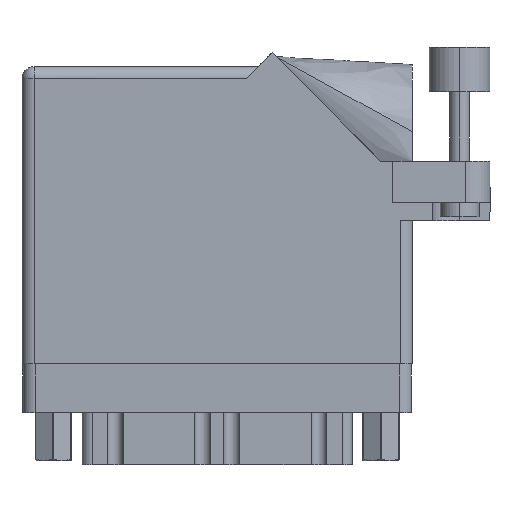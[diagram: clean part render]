
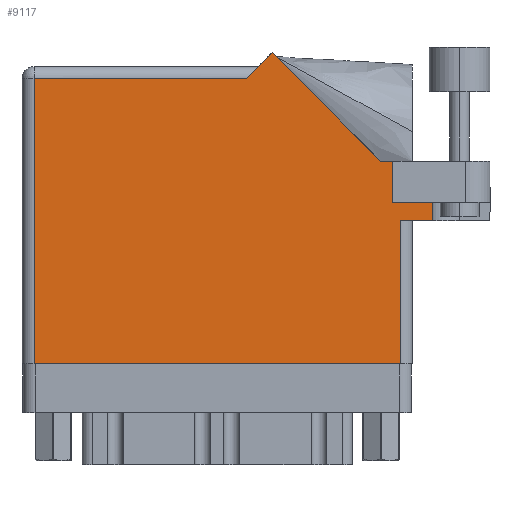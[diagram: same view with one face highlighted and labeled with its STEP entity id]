
A CAD part, front view. The second image highlights one B-rep face of the part: STEP entity #9117.
In plain terms, the highlighted face is planar.
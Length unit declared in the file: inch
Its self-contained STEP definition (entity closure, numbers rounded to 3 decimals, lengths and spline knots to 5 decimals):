
#818 = ORIENTED_EDGE ( 'NONE', *, *, #22465, .T. ) ;
#1750 = FACE_OUTER_BOUND ( 'NONE', #42645, .T. ) ;
#2393 = ORIENTED_EDGE ( 'NONE', *, *, #38100, .T. ) ;
#2926 = CARTESIAN_POINT ( 'NONE',  ( 1.948, 0.737, 0. ) ) ;
#2951 = VERTEX_POINT ( 'NONE', #8101 ) ;
#3372 = LINE ( 'NONE', #7256, #15728 ) ;
#3553 = VERTEX_POINT ( 'NONE', #5469 ) ;
#4420 = EDGE_CURVE ( 'NONE', #41821, #39390, #45638, .T. ) ;
#4458 = VECTOR ( 'NONE', #14354, 39.37008 ) ;
#4657 = CARTESIAN_POINT ( 'NONE',  ( 1.948, 0.737, 0. ) ) ;
#5469 = CARTESIAN_POINT ( 'NONE',  ( 1.91, 1.044, 0. ) ) ;
#5894 = EDGE_CURVE ( 'NONE', #24970, #6006, #18654, .T. ) ;
#6006 = VERTEX_POINT ( 'NONE', #43447 ) ;
#6350 = EDGE_CURVE ( 'NONE', #17928, #39390, #37584, .T. ) ;
#6385 = VECTOR ( 'NONE', #17663, 39.37008 ) ;
#7256 = CARTESIAN_POINT ( 'NONE',  ( 1.84442, 1.044, 0. ) ) ;
#7576 = LINE ( 'NONE', #33860, #27539 ) ;
#8101 = CARTESIAN_POINT ( 'NONE',  ( 1.91, 0.831, 0. ) ) ;
#8550 = ORIENTED_EDGE ( 'NONE', *, *, #29439, .T. ) ;
#9117 = ADVANCED_FACE ( 'NONE', ( #1750 ), #26861, .F. ) ;
#9254 = CARTESIAN_POINT ( 'NONE',  ( 0., 1.468, 0. ) ) ;
#9291 = CARTESIAN_POINT ( 'NONE',  ( 1.91, 0.831, 0. ) ) ;
#10376 = CARTESIAN_POINT ( 'NONE',  ( 2.1115, 0.737, 0. ) ) ;
#10436 = CARTESIAN_POINT ( 'NONE',  ( 1.84442, 1.044, 0. ) ) ;
#13800 = VECTOR ( 'NONE', #30621, 39.37008 ) ;
#14354 = DIRECTION ( 'NONE',  ( -0.707, -0.707, 0. ) ) ;
#15728 = VECTOR ( 'NONE', #18330, 39.37008 ) ;
#16758 = CARTESIAN_POINT ( 'NONE',  ( 0.062, 1.468, 0. ) ) ;
#17663 = DIRECTION ( 'NONE',  ( 0., 1., 0. ) ) ;
#17928 = VERTEX_POINT ( 'NONE', #23054 ) ;
#18197 = LINE ( 'NONE', #39715, #4458 ) ;
#18330 = DIRECTION ( 'NONE',  ( -0.707, 0.707, 0. ) ) ;
#18363 = VECTOR ( 'NONE', #45810, 39.37008 ) ;
#18483 = ORIENTED_EDGE ( 'NONE', *, *, #25661, .T. ) ;
#18531 = ORIENTED_EDGE ( 'NONE', *, *, #46637, .F. ) ;
#18654 = LINE ( 'NONE', #19109, #40227 ) ;
#19109 = CARTESIAN_POINT ( 'NONE',  ( 0.062, 0., 0. ) ) ;
#19128 = VECTOR ( 'NONE', #41120, 39.37008 ) ;
#19807 = EDGE_CURVE ( 'NONE', #6006, #39702, #22893, .T. ) ;
#20011 = ORIENTED_EDGE ( 'NONE', *, *, #28339, .T. ) ;
#21288 = LINE ( 'NONE', #2926, #6385 ) ;
#22444 = VERTEX_POINT ( 'NONE', #10436 ) ;
#22465 = EDGE_CURVE ( 'NONE', #39702, #41821, #21288, .T. ) ;
#22553 = CARTESIAN_POINT ( 'NONE',  ( 1.155, 1.468, 0. ) ) ;
#22893 = LINE ( 'NONE', #27870, #30892 ) ;
#22985 = DIRECTION ( 'NONE',  ( -1., 0., 0. ) ) ;
#23054 = CARTESIAN_POINT ( 'NONE',  ( 2.1115, 0.831, 0. ) ) ;
#23489 = CARTESIAN_POINT ( 'NONE',  ( 0., 1.53, 0. ) ) ;
#24970 = VERTEX_POINT ( 'NONE', #16758 ) ;
#25661 = EDGE_CURVE ( 'NONE', #22444, #30979, #3372, .T. ) ;
#25955 = VECTOR ( 'NONE', #38731, 39.37008 ) ;
#26861 = PLANE ( 'NONE',  #30449 ) ;
#27112 = LINE ( 'NONE', #9254, #38054 ) ;
#27249 = ORIENTED_EDGE ( 'NONE', *, *, #5894, .T. ) ;
#27539 = VECTOR ( 'NONE', #22985, 39.37008 ) ;
#27870 = CARTESIAN_POINT ( 'NONE',  ( 0., 0., 0. ) ) ;
#28072 = EDGE_CURVE ( 'NONE', #2951, #3553, #42371, .T. ) ;
#28339 = EDGE_CURVE ( 'NONE', #3553, #22444, #7576, .T. ) ;
#29439 = EDGE_CURVE ( 'NONE', #30979, #45031, #18197, .T. ) ;
#30449 = AXIS2_PLACEMENT_3D ( 'NONE', #23489, #45952, #41614 ) ;
#30621 = DIRECTION ( 'NONE',  ( 1., 0., 0. ) ) ;
#30892 = VECTOR ( 'NONE', #42628, 39.37008 ) ;
#30979 = VERTEX_POINT ( 'NONE', #45438 ) ;
#31206 = DIRECTION ( 'NONE',  ( -1., 0., 0. ) ) ;
#32939 = ORIENTED_EDGE ( 'NONE', *, *, #4420, .T. ) ;
#33390 = LINE ( 'NONE', #44509, #19128 ) ;
#33782 = CARTESIAN_POINT ( 'NONE',  ( 2.01, 0.737, 0. ) ) ;
#33860 = CARTESIAN_POINT ( 'NONE',  ( 2.41, 1.044, 0. ) ) ;
#34485 = ORIENTED_EDGE ( 'NONE', *, *, #6350, .F. ) ;
#36010 = ORIENTED_EDGE ( 'NONE', *, *, #28072, .T. ) ;
#37001 = DIRECTION ( 'NONE',  ( 0., -1., 0. ) ) ;
#37584 = LINE ( 'NONE', #44864, #18363 ) ;
#37623 = CARTESIAN_POINT ( 'NONE',  ( 1.948, 0., 0. ) ) ;
#38054 = VECTOR ( 'NONE', #31206, 39.37008 ) ;
#38100 = EDGE_CURVE ( 'NONE', #45031, #24970, #27112, .T. ) ;
#38731 = DIRECTION ( 'NONE',  ( 0., 1., 0. ) ) ;
#39012 = ORIENTED_EDGE ( 'NONE', *, *, #19807, .T. ) ;
#39390 = VERTEX_POINT ( 'NONE', #10376 ) ;
#39702 = VERTEX_POINT ( 'NONE', #37623 ) ;
#39715 = CARTESIAN_POINT ( 'NONE',  ( 1.217, 1.53, 0. ) ) ;
#40227 = VECTOR ( 'NONE', #37001, 39.37008 ) ;
#41120 = DIRECTION ( 'NONE',  ( 1., 0., 0. ) ) ;
#41614 = DIRECTION ( 'NONE',  ( -1., 0., 0. ) ) ;
#41821 = VERTEX_POINT ( 'NONE', #4657 ) ;
#42371 = LINE ( 'NONE', #9291, #25955 ) ;
#42628 = DIRECTION ( 'NONE',  ( 1., 0., 0. ) ) ;
#42645 = EDGE_LOOP ( 'NONE', ( #39012, #818, #32939, #34485, #18531, #36010, #20011, #18483, #8550, #2393, #27249 ) ) ;
#43447 = CARTESIAN_POINT ( 'NONE',  ( 0.062, 0., 0. ) ) ;
#44509 = CARTESIAN_POINT ( 'NONE',  ( 1.91, 0.831, 0. ) ) ;
#44864 = CARTESIAN_POINT ( 'NONE',  ( 2.1115, 1.16177, 0. ) ) ;
#45031 = VERTEX_POINT ( 'NONE', #22553 ) ;
#45438 = CARTESIAN_POINT ( 'NONE',  ( 1.28771, 1.60071, 0. ) ) ;
#45638 = LINE ( 'NONE', #33782, #13800 ) ;
#45810 = DIRECTION ( 'NONE',  ( 0., -1., 0. ) ) ;
#45952 = DIRECTION ( 'NONE',  ( 0., 0., -1. ) ) ;
#46637 = EDGE_CURVE ( 'NONE', #2951, #17928, #33390, .T. ) ;
